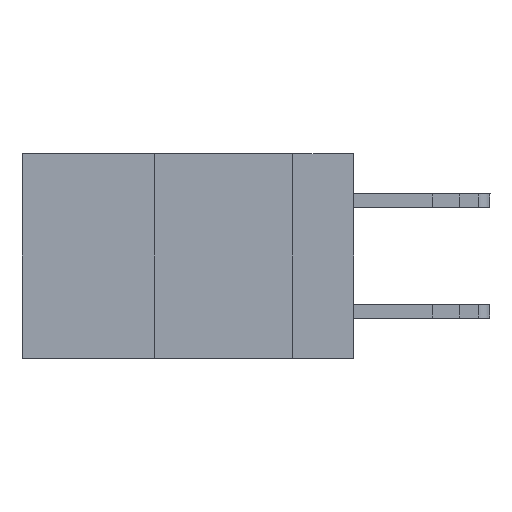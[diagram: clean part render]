
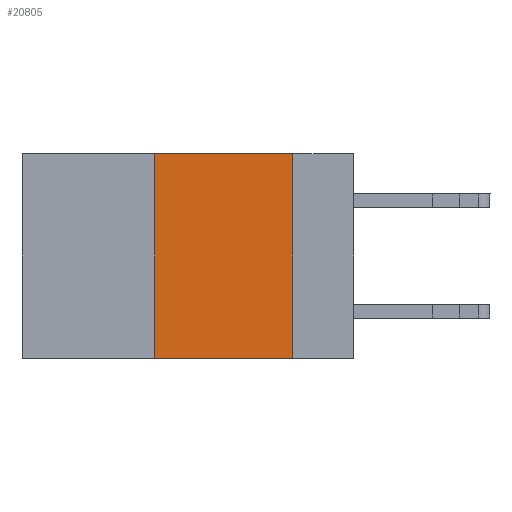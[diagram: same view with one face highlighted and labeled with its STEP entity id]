
A CAD part, left-side view. The second image highlights one B-rep face of the part: STEP entity #20805.
In plain terms, the highlighted planar face has unit normal (-1, 0, 0).
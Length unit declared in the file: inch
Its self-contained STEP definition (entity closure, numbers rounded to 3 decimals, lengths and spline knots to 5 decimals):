
#571 = ORIENTED_EDGE ( 'NONE', *, *, #5232, .F. ) ;
#776 = VERTEX_POINT ( 'NONE', #1800 ) ;
#1134 = EDGE_LOOP ( 'NONE', ( #571, #7703, #10395, #10290 ) ) ;
#1435 = VECTOR ( 'NONE', #26286, 39.37008 ) ;
#1507 = DIRECTION ( 'NONE',  ( 0., 0., -1. ) ) ;
#1800 = CARTESIAN_POINT ( 'NONE',  ( 0., 0.11, 0. ) ) ;
#3590 = EDGE_CURVE ( 'NONE', #20735, #776, #25967, .T. ) ;
#5232 = EDGE_CURVE ( 'NONE', #776, #28719, #18172, .T. ) ;
#7703 = ORIENTED_EDGE ( 'NONE', *, *, #3590, .F. ) ;
#7840 = CARTESIAN_POINT ( 'NONE',  ( 0., 0.36, -0.37 ) ) ;
#7906 = CARTESIAN_POINT ( 'NONE',  ( 0., 0.36, 0. ) ) ;
#8628 = AXIS2_PLACEMENT_3D ( 'NONE', #30649, #12027, #8998 ) ;
#8998 = DIRECTION ( 'NONE',  ( 0., 0., -1. ) ) ;
#9295 = VECTOR ( 'NONE', #25679, 39.37008 ) ;
#10290 = ORIENTED_EDGE ( 'NONE', *, *, #27203, .T. ) ;
#10395 = ORIENTED_EDGE ( 'NONE', *, *, #28382, .F. ) ;
#11475 = CARTESIAN_POINT ( 'NONE',  ( 0., 0.36, 0. ) ) ;
#12027 = DIRECTION ( 'NONE',  ( 1., 0., 0. ) ) ;
#12498 = LINE ( 'NONE', #30486, #24796 ) ;
#14144 = PLANE ( 'NONE',  #8628 ) ;
#14523 = CARTESIAN_POINT ( 'NONE',  ( 0., 0.6, 0. ) ) ;
#16061 = LINE ( 'NONE', #11475, #9295 ) ;
#18172 = LINE ( 'NONE', #34346, #27560 ) ;
#20735 = VERTEX_POINT ( 'NONE', #7906 ) ;
#20805 = ADVANCED_FACE ( 'NONE', ( #27535 ), #14144, .F. ) ;
#24796 = VECTOR ( 'NONE', #31096, 39.37008 ) ;
#25679 = DIRECTION ( 'NONE',  ( 0., 0., 1. ) ) ;
#25967 = LINE ( 'NONE', #14523, #1435 ) ;
#26185 = VERTEX_POINT ( 'NONE', #7840 ) ;
#26286 = DIRECTION ( 'NONE',  ( 0., -1., 0. ) ) ;
#27203 = EDGE_CURVE ( 'NONE', #26185, #28719, #12498, .T. ) ;
#27535 = FACE_OUTER_BOUND ( 'NONE', #1134, .T. ) ;
#27560 = VECTOR ( 'NONE', #1507, 39.37008 ) ;
#28382 = EDGE_CURVE ( 'NONE', #26185, #20735, #16061, .T. ) ;
#28719 = VERTEX_POINT ( 'NONE', #31944 ) ;
#30486 = CARTESIAN_POINT ( 'NONE',  ( 0., 0.6, -0.37 ) ) ;
#30649 = CARTESIAN_POINT ( 'NONE',  ( 0., 0.6, 0. ) ) ;
#31096 = DIRECTION ( 'NONE',  ( 0., -1., 0. ) ) ;
#31944 = CARTESIAN_POINT ( 'NONE',  ( 0., 0.11, -0.37 ) ) ;
#34346 = CARTESIAN_POINT ( 'NONE',  ( 0., 0.11, 0. ) ) ;
